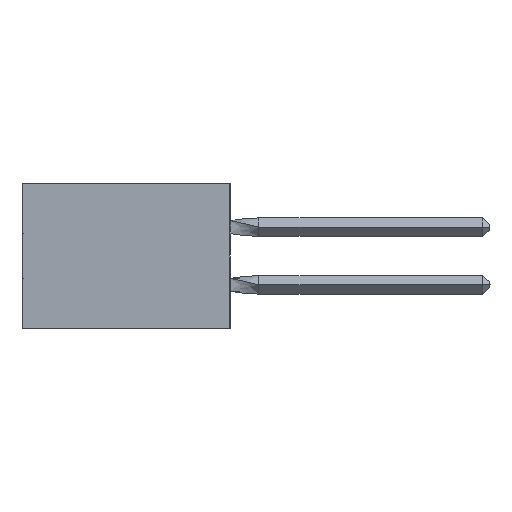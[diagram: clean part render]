
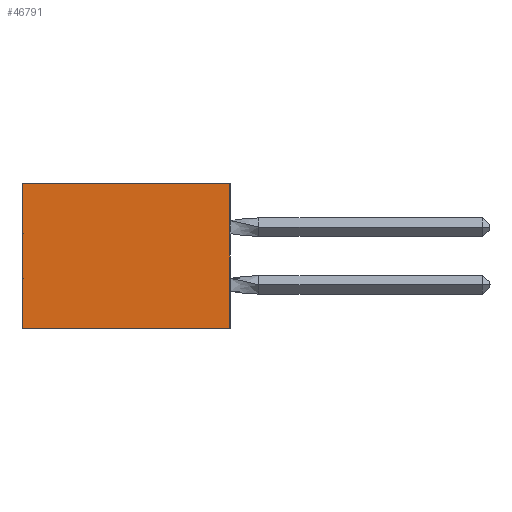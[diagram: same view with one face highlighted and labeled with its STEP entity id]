
A CAD part, left-side view. The second image highlights one B-rep face of the part: STEP entity #46791.
In plain terms, the highlighted planar face has unit normal (-1, 0, 0).
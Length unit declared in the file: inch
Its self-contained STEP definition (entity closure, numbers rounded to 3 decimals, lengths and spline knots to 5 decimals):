
#1029 = EDGE_LOOP ( 'NONE', ( #9351, #42988, #5864, #31286 ) ) ;
#2352 = CARTESIAN_POINT ( 'NONE',  ( 0.305, 0.72, -0.5 ) ) ;
#2679 = DIRECTION ( 'NONE',  ( 0., 0., -1. ) ) ;
#5864 = ORIENTED_EDGE ( 'NONE', *, *, #43934, .F. ) ;
#7430 = CARTESIAN_POINT ( 'NONE',  ( 0.305, 0., -0.5 ) ) ;
#7481 = CARTESIAN_POINT ( 'NONE',  ( 0.305, 0.72, 0. ) ) ;
#8254 = FACE_OUTER_BOUND ( 'NONE', #1029, .T. ) ;
#8798 = CARTESIAN_POINT ( 'NONE',  ( 0.305, 0., -0.5 ) ) ;
#9351 = ORIENTED_EDGE ( 'NONE', *, *, #35738, .T. ) ;
#13066 = EDGE_CURVE ( 'NONE', #22591, #23999, #19764, .T. ) ;
#13568 = VECTOR ( 'NONE', #2679, 39.37008 ) ;
#14517 = DIRECTION ( 'NONE',  ( 0., 1., 0. ) ) ;
#15549 = CARTESIAN_POINT ( 'NONE',  ( 0.305, 0., 0. ) ) ;
#16413 = CARTESIAN_POINT ( 'NONE',  ( 0.305, 0., -0.5 ) ) ;
#16520 = VERTEX_POINT ( 'NONE', #15549 ) ;
#17536 = LINE ( 'NONE', #38957, #13568 ) ;
#17592 = CARTESIAN_POINT ( 'NONE',  ( 0.305, 0., -0.5 ) ) ;
#19092 = VECTOR ( 'NONE', #34159, 39.37008 ) ;
#19764 = LINE ( 'NONE', #8798, #20947 ) ;
#20947 = VECTOR ( 'NONE', #45447, 39.37008 ) ;
#22591 = VERTEX_POINT ( 'NONE', #17592 ) ;
#23999 = VERTEX_POINT ( 'NONE', #2352 ) ;
#24835 = LINE ( 'NONE', #16413, #19092 ) ;
#25607 = VECTOR ( 'NONE', #14517, 39.37008 ) ;
#29240 = PLANE ( 'NONE',  #40877 ) ;
#31286 = ORIENTED_EDGE ( 'NONE', *, *, #34821, .T. ) ;
#32946 = DIRECTION ( 'NONE',  ( 1., 0., 0. ) ) ;
#34159 = DIRECTION ( 'NONE',  ( 0., 0., -1. ) ) ;
#34220 = VERTEX_POINT ( 'NONE', #7481 ) ;
#34821 = EDGE_CURVE ( 'NONE', #16520, #34220, #39801, .T. ) ;
#35738 = EDGE_CURVE ( 'NONE', #34220, #23999, #17536, .T. ) ;
#36532 = DIRECTION ( 'NONE',  ( 0., 0., -1. ) ) ;
#38321 = CARTESIAN_POINT ( 'NONE',  ( 0.305, 0., 0. ) ) ;
#38957 = CARTESIAN_POINT ( 'NONE',  ( 0.305, 0.72, -0.5 ) ) ;
#39801 = LINE ( 'NONE', #38321, #25607 ) ;
#40877 = AXIS2_PLACEMENT_3D ( 'NONE', #7430, #32946, #36532 ) ;
#42988 = ORIENTED_EDGE ( 'NONE', *, *, #13066, .F. ) ;
#43934 = EDGE_CURVE ( 'NONE', #16520, #22591, #24835, .T. ) ;
#45447 = DIRECTION ( 'NONE',  ( 0., 1., 0. ) ) ;
#46791 = ADVANCED_FACE ( 'NONE', ( #8254 ), #29240, .F. ) ;
